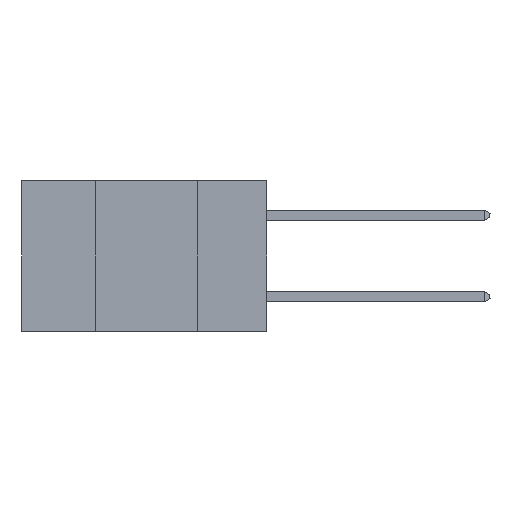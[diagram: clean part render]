
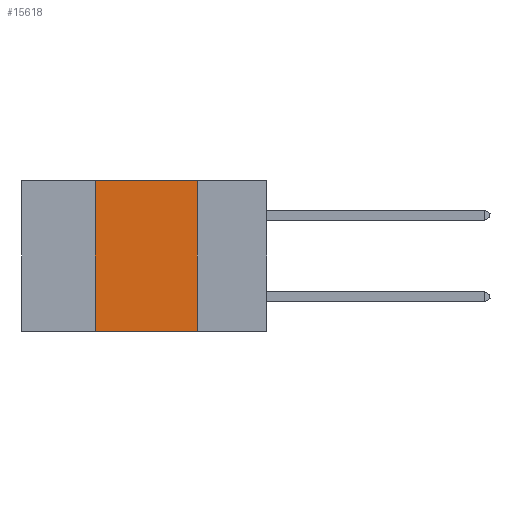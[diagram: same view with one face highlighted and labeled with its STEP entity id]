
A CAD part, left-side view. The second image highlights one B-rep face of the part: STEP entity #15618.
In plain terms, the highlighted planar face has unit normal (-1, 0, 0).
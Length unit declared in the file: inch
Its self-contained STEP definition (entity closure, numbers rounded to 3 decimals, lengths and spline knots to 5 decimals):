
#910 = CARTESIAN_POINT ( 'NONE',  ( 0., 0.6, 0. ) ) ;
#1351 = AXIS2_PLACEMENT_3D ( 'NONE', #910, #3066, #17430 ) ;
#1374 = LINE ( 'NONE', #11503, #21915 ) ;
#2475 = VECTOR ( 'NONE', #5585, 39.37008 ) ;
#3066 = DIRECTION ( 'NONE',  ( 1., 0., 0. ) ) ;
#3205 = DIRECTION ( 'NONE',  ( 0., -1., 0. ) ) ;
#4044 = CARTESIAN_POINT ( 'NONE',  ( 0., 0.6, -0.37 ) ) ;
#4253 = CARTESIAN_POINT ( 'NONE',  ( 0., 0.42, -0.37 ) ) ;
#5119 = VECTOR ( 'NONE', #3205, 39.37008 ) ;
#5585 = DIRECTION ( 'NONE',  ( 0., 0., -1. ) ) ;
#6832 = EDGE_LOOP ( 'NONE', ( #9856, #21250, #6950, #17791 ) ) ;
#6950 = ORIENTED_EDGE ( 'NONE', *, *, #8624, .F. ) ;
#6956 = VERTEX_POINT ( 'NONE', #4253 ) ;
#7609 = CARTESIAN_POINT ( 'NONE',  ( 0., 0.17, -0.37 ) ) ;
#8624 = EDGE_CURVE ( 'NONE', #6956, #9476, #1374, .T. ) ;
#9476 = VERTEX_POINT ( 'NONE', #19997 ) ;
#9856 = ORIENTED_EDGE ( 'NONE', *, *, #14649, .F. ) ;
#11503 = CARTESIAN_POINT ( 'NONE',  ( 0., 0.42, 0. ) ) ;
#11507 = CARTESIAN_POINT ( 'NONE',  ( 0., 0.6, 0. ) ) ;
#14539 = EDGE_CURVE ( 'NONE', #9476, #16007, #21389, .T. ) ;
#14542 = CARTESIAN_POINT ( 'NONE',  ( 0., 0.17, 0. ) ) ;
#14649 = EDGE_CURVE ( 'NONE', #16007, #23776, #24214, .T. ) ;
#15444 = PLANE ( 'NONE',  #1351 ) ;
#15618 = ADVANCED_FACE ( 'NONE', ( #17973 ), #15444, .F. ) ;
#15834 = CARTESIAN_POINT ( 'NONE',  ( 0., 0.17, 0. ) ) ;
#16007 = VERTEX_POINT ( 'NONE', #14542 ) ;
#16898 = VECTOR ( 'NONE', #24357, 39.37008 ) ;
#17430 = DIRECTION ( 'NONE',  ( 0., 0., -1. ) ) ;
#17791 = ORIENTED_EDGE ( 'NONE', *, *, #17904, .T. ) ;
#17904 = EDGE_CURVE ( 'NONE', #6956, #23776, #22245, .T. ) ;
#17973 = FACE_OUTER_BOUND ( 'NONE', #6832, .T. ) ;
#19997 = CARTESIAN_POINT ( 'NONE',  ( 0., 0.42, 0. ) ) ;
#21250 = ORIENTED_EDGE ( 'NONE', *, *, #14539, .F. ) ;
#21389 = LINE ( 'NONE', #11507, #5119 ) ;
#21915 = VECTOR ( 'NONE', #23561, 39.37008 ) ;
#22245 = LINE ( 'NONE', #4044, #16898 ) ;
#23561 = DIRECTION ( 'NONE',  ( 0., 0., 1. ) ) ;
#23776 = VERTEX_POINT ( 'NONE', #7609 ) ;
#24214 = LINE ( 'NONE', #15834, #2475 ) ;
#24357 = DIRECTION ( 'NONE',  ( 0., -1., 0. ) ) ;
